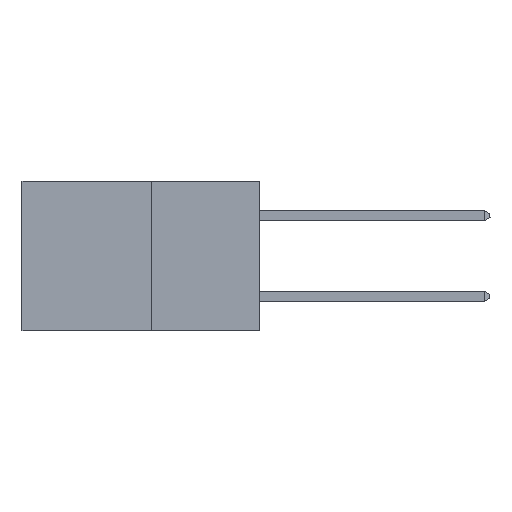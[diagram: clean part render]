
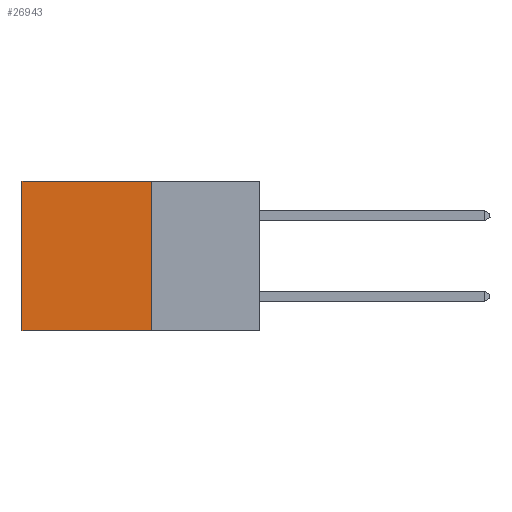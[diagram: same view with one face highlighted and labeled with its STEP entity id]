
A CAD part, left-side view. The second image highlights one B-rep face of the part: STEP entity #26943.
In plain terms, the highlighted planar face has unit normal (-1, 0, 0).
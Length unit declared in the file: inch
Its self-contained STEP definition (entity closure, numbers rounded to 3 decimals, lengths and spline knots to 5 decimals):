
#344 = EDGE_LOOP ( 'NONE', ( #6146, #11253, #4585, #16038 ) ) ;
#964 = AXIS2_PLACEMENT_3D ( 'NONE', #2911, #5660, #24398 ) ;
#2547 = CARTESIAN_POINT ( 'NONE',  ( 0.277, 0.27, 0. ) ) ;
#2911 = CARTESIAN_POINT ( 'NONE',  ( 0.277, 0.27, -0.37 ) ) ;
#3211 = CARTESIAN_POINT ( 'NONE',  ( 0.277, 0.59, 0. ) ) ;
#3578 = VERTEX_POINT ( 'NONE', #3211 ) ;
#4585 = ORIENTED_EDGE ( 'NONE', *, *, #14183, .F. ) ;
#5660 = DIRECTION ( 'NONE',  ( 1., 0., 0. ) ) ;
#6146 = ORIENTED_EDGE ( 'NONE', *, *, #7339, .T. ) ;
#7339 = EDGE_CURVE ( 'NONE', #3578, #29519, #18347, .T. ) ;
#7708 = CARTESIAN_POINT ( 'NONE',  ( 0.277, 0.27, -0.37 ) ) ;
#10436 = VECTOR ( 'NONE', #21407, 39.37008 ) ;
#11253 = ORIENTED_EDGE ( 'NONE', *, *, #13024, .F. ) ;
#11413 = CARTESIAN_POINT ( 'NONE',  ( 0.277, 0.27, -0.37 ) ) ;
#13024 = EDGE_CURVE ( 'NONE', #29307, #29519, #21505, .T. ) ;
#13510 = VECTOR ( 'NONE', #32456, 39.37008 ) ;
#13847 = LINE ( 'NONE', #7708, #25491 ) ;
#14183 = EDGE_CURVE ( 'NONE', #25727, #29307, #13847, .T. ) ;
#16038 = ORIENTED_EDGE ( 'NONE', *, *, #24416, .T. ) ;
#18347 = LINE ( 'NONE', #33963, #24578 ) ;
#18738 = CARTESIAN_POINT ( 'NONE',  ( 0.277, 0.59, -0.37 ) ) ;
#19078 = PLANE ( 'NONE',  #964 ) ;
#21113 = DIRECTION ( 'NONE',  ( 0., 0., -1. ) ) ;
#21407 = DIRECTION ( 'NONE',  ( 0., 1., 0. ) ) ;
#21505 = LINE ( 'NONE', #11413, #13510 ) ;
#22240 = CARTESIAN_POINT ( 'NONE',  ( 0.277, 0.27, 0. ) ) ;
#24398 = DIRECTION ( 'NONE',  ( 0., 0., -1. ) ) ;
#24416 = EDGE_CURVE ( 'NONE', #25727, #3578, #30687, .T. ) ;
#24578 = VECTOR ( 'NONE', #33608, 39.37008 ) ;
#25228 = FACE_OUTER_BOUND ( 'NONE', #344, .T. ) ;
#25491 = VECTOR ( 'NONE', #21113, 39.37008 ) ;
#25727 = VERTEX_POINT ( 'NONE', #22240 ) ;
#26943 = ADVANCED_FACE ( 'NONE', ( #25228 ), #19078, .F. ) ;
#27903 = CARTESIAN_POINT ( 'NONE',  ( 0.277, 0.27, -0.37 ) ) ;
#29307 = VERTEX_POINT ( 'NONE', #27903 ) ;
#29519 = VERTEX_POINT ( 'NONE', #18738 ) ;
#30687 = LINE ( 'NONE', #2547, #10436 ) ;
#32456 = DIRECTION ( 'NONE',  ( 0., 1., 0. ) ) ;
#33608 = DIRECTION ( 'NONE',  ( 0., 0., -1. ) ) ;
#33963 = CARTESIAN_POINT ( 'NONE',  ( 0.277, 0.59, -0.37 ) ) ;
